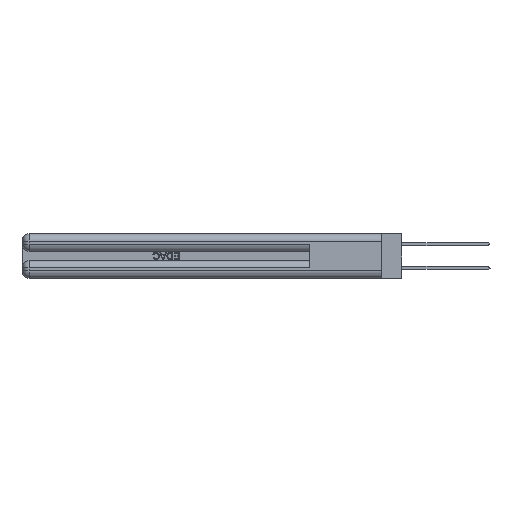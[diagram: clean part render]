
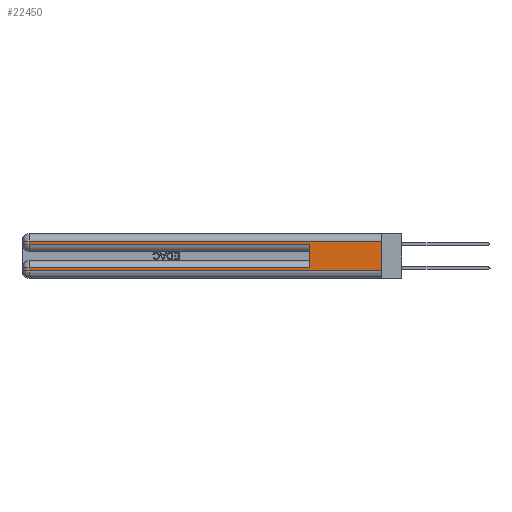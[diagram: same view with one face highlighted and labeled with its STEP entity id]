
A CAD part, left-side view. The second image highlights one B-rep face of the part: STEP entity #22450.
In plain terms, the highlighted planar face has unit normal (-1, 0, 0).
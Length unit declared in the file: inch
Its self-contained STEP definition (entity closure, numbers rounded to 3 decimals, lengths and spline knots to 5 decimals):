
#787 = AXIS2_PLACEMENT_3D ( 'NONE', #11654, #24754, #15043 ) ;
#800 = VERTEX_POINT ( 'NONE', #7842 ) ;
#1308 = LINE ( 'NONE', #40310, #3376 ) ;
#2461 = ORIENTED_EDGE ( 'NONE', *, *, #37154, .T. ) ;
#3005 = EDGE_CURVE ( 'NONE', #800, #33995, #17773, .T. ) ;
#3376 = VECTOR ( 'NONE', #8354, 39.37008 ) ;
#4098 = LINE ( 'NONE', #28328, #19828 ) ;
#5564 = PLANE ( 'NONE',  #787 ) ;
#6820 = ORIENTED_EDGE ( 'NONE', *, *, #29033, .T. ) ;
#7710 = VECTOR ( 'NONE', #13614, 39.37008 ) ;
#7842 = CARTESIAN_POINT ( 'NONE',  ( 0., 0., 0.31 ) ) ;
#8354 = DIRECTION ( 'NONE',  ( 0., 0., -1. ) ) ;
#8625 = EDGE_CURVE ( 'NONE', #800, #9239, #1308, .T. ) ;
#8805 = EDGE_CURVE ( 'NONE', #33995, #33068, #34523, .T. ) ;
#9167 = VECTOR ( 'NONE', #14210, 39.37008 ) ;
#9226 = LINE ( 'NONE', #33197, #7710 ) ;
#9239 = VERTEX_POINT ( 'NONE', #17048 ) ;
#9318 = CARTESIAN_POINT ( 'NONE',  ( 0., 2.94, 0.085 ) ) ;
#9685 = ORIENTED_EDGE ( 'NONE', *, *, #21779, .F. ) ;
#11654 = CARTESIAN_POINT ( 'NONE',  ( 0., 0., 0.37 ) ) ;
#12110 = VECTOR ( 'NONE', #16507, 39.37008 ) ;
#12586 = VERTEX_POINT ( 'NONE', #16813 ) ;
#13614 = DIRECTION ( 'NONE',  ( 0., 0., -1. ) ) ;
#14210 = DIRECTION ( 'NONE',  ( 0., 1., 0. ) ) ;
#15043 = DIRECTION ( 'NONE',  ( 0., 0., -1. ) ) ;
#15326 = DIRECTION ( 'NONE',  ( 0., 1., 0. ) ) ;
#16216 = LINE ( 'NONE', #39081, #12110 ) ;
#16507 = DIRECTION ( 'NONE',  ( 0., 0., 1. ) ) ;
#16813 = CARTESIAN_POINT ( 'NONE',  ( 0., 2.94, 0.06 ) ) ;
#17048 = CARTESIAN_POINT ( 'NONE',  ( 0., 0., 0.06 ) ) ;
#17064 = VECTOR ( 'NONE', #40959, 39.37008 ) ;
#17773 = LINE ( 'NONE', #37480, #9167 ) ;
#18085 = VERTEX_POINT ( 'NONE', #9318 ) ;
#18731 = LINE ( 'NONE', #23886, #20764 ) ;
#19828 = VECTOR ( 'NONE', #15326, 39.37008 ) ;
#20764 = VECTOR ( 'NONE', #33622, 39.37008 ) ;
#21779 = EDGE_CURVE ( 'NONE', #26955, #30631, #16216, .T. ) ;
#22248 = EDGE_CURVE ( 'NONE', #12586, #9239, #23316, .T. ) ;
#22450 = ADVANCED_FACE ( 'NONE', ( #29937 ), #5564, .F. ) ;
#23316 = LINE ( 'NONE', #29510, #40187 ) ;
#23744 = ORIENTED_EDGE ( 'NONE', *, *, #3005, .T. ) ;
#23886 = CARTESIAN_POINT ( 'NONE',  ( 0., 0., 0.285 ) ) ;
#24335 = CARTESIAN_POINT ( 'NONE',  ( 0., 2.94, 0.37 ) ) ;
#24754 = DIRECTION ( 'NONE',  ( 1., 0., 0. ) ) ;
#25245 = CARTESIAN_POINT ( 'NONE',  ( 0., 2.94, 0.31 ) ) ;
#26326 = ORIENTED_EDGE ( 'NONE', *, *, #32498, .T. ) ;
#26623 = ORIENTED_EDGE ( 'NONE', *, *, #8625, .F. ) ;
#26955 = VERTEX_POINT ( 'NONE', #38493 ) ;
#28328 = CARTESIAN_POINT ( 'NONE',  ( 0., 0., 0.085 ) ) ;
#29033 = EDGE_CURVE ( 'NONE', #18085, #12586, #9226, .T. ) ;
#29510 = CARTESIAN_POINT ( 'NONE',  ( 0., 0., 0.06 ) ) ;
#29937 = FACE_OUTER_BOUND ( 'NONE', #39094, .T. ) ;
#30631 = VERTEX_POINT ( 'NONE', #41196 ) ;
#32498 = EDGE_CURVE ( 'NONE', #33068, #30631, #18731, .T. ) ;
#33068 = VERTEX_POINT ( 'NONE', #40474 ) ;
#33197 = CARTESIAN_POINT ( 'NONE',  ( 0., 2.94, 0.37 ) ) ;
#33622 = DIRECTION ( 'NONE',  ( 0., -1., 0. ) ) ;
#33995 = VERTEX_POINT ( 'NONE', #25245 ) ;
#34222 = ORIENTED_EDGE ( 'NONE', *, *, #8805, .T. ) ;
#34523 = LINE ( 'NONE', #24335, #17064 ) ;
#36379 = DIRECTION ( 'NONE',  ( 0., -1., 0. ) ) ;
#37154 = EDGE_CURVE ( 'NONE', #26955, #18085, #4098, .T. ) ;
#37480 = CARTESIAN_POINT ( 'NONE',  ( 0., 0., 0.31 ) ) ;
#38493 = CARTESIAN_POINT ( 'NONE',  ( 0., 0.6, 0.085 ) ) ;
#39081 = CARTESIAN_POINT ( 'NONE',  ( 0., 0.6, 0.145 ) ) ;
#39094 = EDGE_LOOP ( 'NONE', ( #26623, #23744, #34222, #26326, #9685, #2461, #6820, #41416 ) ) ;
#40187 = VECTOR ( 'NONE', #36379, 39.37008 ) ;
#40310 = CARTESIAN_POINT ( 'NONE',  ( 0., 0., 0.37 ) ) ;
#40474 = CARTESIAN_POINT ( 'NONE',  ( 0., 2.94, 0.285 ) ) ;
#40959 = DIRECTION ( 'NONE',  ( 0., 0., -1. ) ) ;
#41196 = CARTESIAN_POINT ( 'NONE',  ( 0., 0.6, 0.285 ) ) ;
#41416 = ORIENTED_EDGE ( 'NONE', *, *, #22248, .T. ) ;
